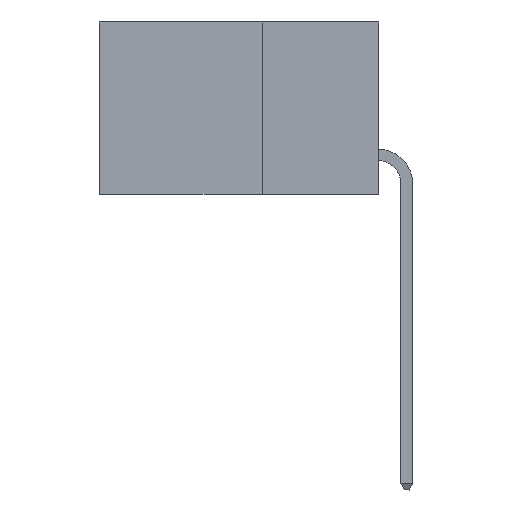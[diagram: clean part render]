
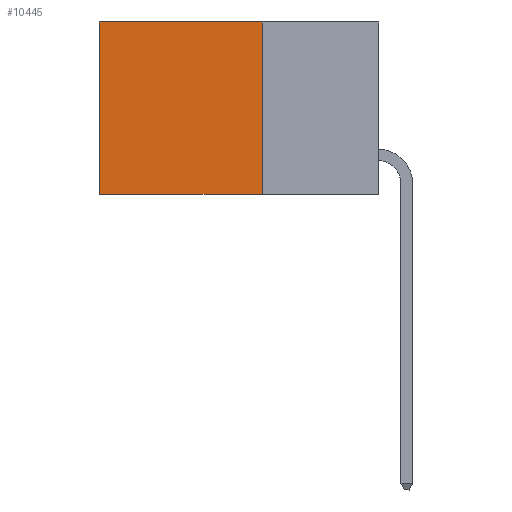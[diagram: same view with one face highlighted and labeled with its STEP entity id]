
A CAD part, left-side view. The second image highlights one B-rep face of the part: STEP entity #10445.
In plain terms, the highlighted planar face has unit normal (-1, 0, 0).
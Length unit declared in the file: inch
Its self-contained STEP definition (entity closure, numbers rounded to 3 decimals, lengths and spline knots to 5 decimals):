
#607 = DIRECTION ( 'NONE',  ( 0., 1., 0. ) ) ;
#1412 = VECTOR ( 'NONE', #16847, 39.37008 ) ;
#1936 = VERTEX_POINT ( 'NONE', #8998 ) ;
#2036 = LINE ( 'NONE', #9518, #5472 ) ;
#2286 = CARTESIAN_POINT ( 'NONE',  ( 0.2615, 0.25, 0. ) ) ;
#2519 = CARTESIAN_POINT ( 'NONE',  ( 0.2615, 0.25, 0. ) ) ;
#2629 = VERTEX_POINT ( 'NONE', #16535 ) ;
#3674 = LINE ( 'NONE', #10968, #1412 ) ;
#3715 = DIRECTION ( 'NONE',  ( 0., 0., -1. ) ) ;
#3802 = DIRECTION ( 'NONE',  ( 1., 0., 0. ) ) ;
#4038 = ORIENTED_EDGE ( 'NONE', *, *, #14180, .F. ) ;
#5472 = VECTOR ( 'NONE', #607, 39.37008 ) ;
#5749 = VERTEX_POINT ( 'NONE', #2519 ) ;
#6294 = LINE ( 'NONE', #2286, #17168 ) ;
#6668 = EDGE_LOOP ( 'NONE', ( #9393, #9167, #4038, #17943 ) ) ;
#6709 = VECTOR ( 'NONE', #13736, 39.37008 ) ;
#7029 = EDGE_CURVE ( 'NONE', #2629, #18114, #3674, .T. ) ;
#8168 = AXIS2_PLACEMENT_3D ( 'NONE', #15274, #3802, #3715 ) ;
#8998 = CARTESIAN_POINT ( 'NONE',  ( 0.2615, 0.25, -0.37 ) ) ;
#9167 = ORIENTED_EDGE ( 'NONE', *, *, #12962, .F. ) ;
#9393 = ORIENTED_EDGE ( 'NONE', *, *, #7029, .T. ) ;
#9518 = CARTESIAN_POINT ( 'NONE',  ( 0.2615, 0.25, -0.37 ) ) ;
#10445 = ADVANCED_FACE ( 'NONE', ( #18415 ), #15559, .F. ) ;
#10968 = CARTESIAN_POINT ( 'NONE',  ( 0.2615, 0.6, -0.37 ) ) ;
#12502 = CARTESIAN_POINT ( 'NONE',  ( 0.2615, 0.25, -0.37 ) ) ;
#12962 = EDGE_CURVE ( 'NONE', #1936, #18114, #2036, .T. ) ;
#13736 = DIRECTION ( 'NONE',  ( 0., 0., -1. ) ) ;
#14180 = EDGE_CURVE ( 'NONE', #5749, #1936, #18195, .T. ) ;
#15274 = CARTESIAN_POINT ( 'NONE',  ( 0.2615, 0.25, -0.37 ) ) ;
#15559 = PLANE ( 'NONE',  #8168 ) ;
#16104 = CARTESIAN_POINT ( 'NONE',  ( 0.2615, 0.6, -0.37 ) ) ;
#16535 = CARTESIAN_POINT ( 'NONE',  ( 0.2615, 0.6, 0. ) ) ;
#16847 = DIRECTION ( 'NONE',  ( 0., 0., -1. ) ) ;
#17168 = VECTOR ( 'NONE', #17862, 39.37008 ) ;
#17862 = DIRECTION ( 'NONE',  ( 0., 1., 0. ) ) ;
#17943 = ORIENTED_EDGE ( 'NONE', *, *, #18731, .T. ) ;
#18114 = VERTEX_POINT ( 'NONE', #16104 ) ;
#18195 = LINE ( 'NONE', #12502, #6709 ) ;
#18415 = FACE_OUTER_BOUND ( 'NONE', #6668, .T. ) ;
#18731 = EDGE_CURVE ( 'NONE', #5749, #2629, #6294, .T. ) ;
